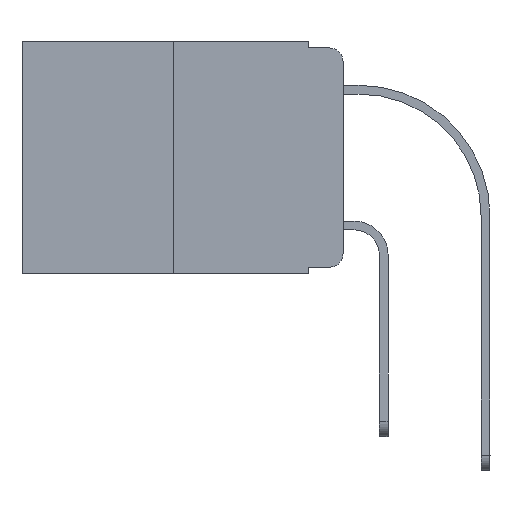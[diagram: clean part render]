
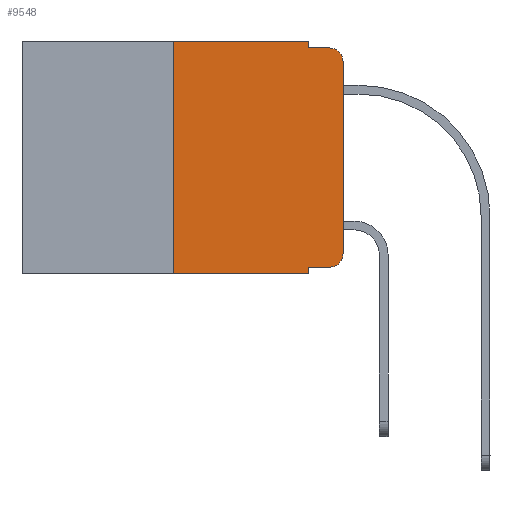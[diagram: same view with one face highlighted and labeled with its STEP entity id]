
A CAD part, left-side view. The second image highlights one B-rep face of the part: STEP entity #9548.
In plain terms, the highlighted planar face has unit normal (-1, 0, 0).
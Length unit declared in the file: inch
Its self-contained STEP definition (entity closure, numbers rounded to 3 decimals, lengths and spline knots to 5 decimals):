
#168 = CARTESIAN_POINT ( 'NONE',  ( 0., 0.02, -0.01 ) ) ;
#239 = VECTOR ( 'NONE', #13982, 39.37008 ) ;
#399 = DIRECTION ( 'NONE',  ( 0., -1., 0. ) ) ;
#440 = ORIENTED_EDGE ( 'NONE', *, *, #2540, .F. ) ;
#729 = EDGE_CURVE ( 'NONE', #20648, #1539, #17899, .T. ) ;
#860 = ORIENTED_EDGE ( 'NONE', *, *, #24218, .F. ) ;
#1041 = ORIENTED_EDGE ( 'NONE', *, *, #22903, .F. ) ;
#1135 = DIRECTION ( 'NONE',  ( 0., -1., 0. ) ) ;
#1462 = ORIENTED_EDGE ( 'NONE', *, *, #11914, .F. ) ;
#1539 = VERTEX_POINT ( 'NONE', #6256 ) ;
#2211 = CARTESIAN_POINT ( 'NONE',  ( 0., 0.051, 0. ) ) ;
#2469 = VECTOR ( 'NONE', #6436, 39.37008 ) ;
#2540 = EDGE_CURVE ( 'NONE', #20648, #21269, #13048, .T. ) ;
#2630 = LINE ( 'NONE', #10619, #2469 ) ;
#2850 = AXIS2_PLACEMENT_3D ( 'NONE', #13515, #21236, #13656 ) ;
#2889 = ORIENTED_EDGE ( 'NONE', *, *, #10489, .T. ) ;
#2893 = LINE ( 'NONE', #4797, #11804 ) ;
#3993 = CARTESIAN_POINT ( 'NONE',  ( 0., 0.25, -0.343 ) ) ;
#4261 = CARTESIAN_POINT ( 'NONE',  ( 0., 0.25, 0. ) ) ;
#4791 = DIRECTION ( 'NONE',  ( 0., 0., -1. ) ) ;
#4797 = CARTESIAN_POINT ( 'NONE',  ( 0., 0.051, -0.01 ) ) ;
#4845 = VERTEX_POINT ( 'NONE', #12068 ) ;
#5395 = LINE ( 'NONE', #16711, #6885 ) ;
#6146 = CIRCLE ( 'NONE', #2850, 0.02 ) ;
#6256 = CARTESIAN_POINT ( 'NONE',  ( 0., 0.02, -0.333 ) ) ;
#6436 = DIRECTION ( 'NONE',  ( 0., -1., 0. ) ) ;
#6885 = VECTOR ( 'NONE', #7432, 39.37008 ) ;
#7432 = DIRECTION ( 'NONE',  ( 0., -1., 0. ) ) ;
#7438 = CARTESIAN_POINT ( 'NONE',  ( 0., 0.25, 0. ) ) ;
#8888 = EDGE_CURVE ( 'NONE', #1539, #14236, #20594, .T. ) ;
#9020 = FACE_OUTER_BOUND ( 'NONE', #10609, .T. ) ;
#9548 = ADVANCED_FACE ( 'NONE', ( #9020 ), #20679, .F. ) ;
#9594 = VERTEX_POINT ( 'NONE', #14889 ) ;
#9600 = DIRECTION ( 'NONE',  ( 0., 0., 1. ) ) ;
#10489 = EDGE_CURVE ( 'NONE', #20383, #21269, #5395, .T. ) ;
#10609 = EDGE_LOOP ( 'NONE', ( #11493, #17040, #1041, #1462, #860, #23297, #2889, #440, #12570, #12920 ) ) ;
#10619 = CARTESIAN_POINT ( 'NONE',  ( 0., 0.473, 0. ) ) ;
#10762 = VERTEX_POINT ( 'NONE', #12007 ) ;
#11179 = CARTESIAN_POINT ( 'NONE',  ( 0., 0.051, -0.343 ) ) ;
#11493 = ORIENTED_EDGE ( 'NONE', *, *, #20991, .T. ) ;
#11804 = VECTOR ( 'NONE', #1135, 39.37008 ) ;
#11822 = CARTESIAN_POINT ( 'NONE',  ( 0., 0., 0. ) ) ;
#11863 = DIRECTION ( 'NONE',  ( -1., 0., 0. ) ) ;
#11914 = EDGE_CURVE ( 'NONE', #10762, #4845, #15546, .T. ) ;
#12007 = CARTESIAN_POINT ( 'NONE',  ( 0., 0.051, 0. ) ) ;
#12068 = CARTESIAN_POINT ( 'NONE',  ( 0., 0.051, -0.01 ) ) ;
#12185 = CARTESIAN_POINT ( 'NONE',  ( 0., 0.051, -0.333 ) ) ;
#12570 = ORIENTED_EDGE ( 'NONE', *, *, #729, .T. ) ;
#12920 = ORIENTED_EDGE ( 'NONE', *, *, #8888, .T. ) ;
#13048 = LINE ( 'NONE', #14845, #15300 ) ;
#13405 = LINE ( 'NONE', #7438, #22323 ) ;
#13515 = CARTESIAN_POINT ( 'NONE',  ( 0., 0.02, -0.03 ) ) ;
#13656 = DIRECTION ( 'NONE',  ( 0., 0., -1. ) ) ;
#13982 = DIRECTION ( 'NONE',  ( 0., 0., 1. ) ) ;
#14236 = VERTEX_POINT ( 'NONE', #16738 ) ;
#14682 = VERTEX_POINT ( 'NONE', #168 ) ;
#14845 = CARTESIAN_POINT ( 'NONE',  ( 0., 0.051, 0. ) ) ;
#14889 = CARTESIAN_POINT ( 'NONE',  ( 0., 0., -0.03 ) ) ;
#15300 = VECTOR ( 'NONE', #4791, 39.37008 ) ;
#15546 = LINE ( 'NONE', #2211, #19998 ) ;
#16711 = CARTESIAN_POINT ( 'NONE',  ( 0., 0.473, -0.343 ) ) ;
#16738 = CARTESIAN_POINT ( 'NONE',  ( 0., 0., -0.313 ) ) ;
#17040 = ORIENTED_EDGE ( 'NONE', *, *, #23680, .T. ) ;
#17714 = CARTESIAN_POINT ( 'NONE',  ( 0., 0.02, -0.313 ) ) ;
#17899 = LINE ( 'NONE', #12185, #24867 ) ;
#19243 = VERTEX_POINT ( 'NONE', #4261 ) ;
#19998 = VECTOR ( 'NONE', #23249, 39.37008 ) ;
#20383 = VERTEX_POINT ( 'NONE', #3993 ) ;
#20594 = CIRCLE ( 'NONE', #21000, 0.02 ) ;
#20648 = VERTEX_POINT ( 'NONE', #23744 ) ;
#20679 = PLANE ( 'NONE',  #21420 ) ;
#20991 = EDGE_CURVE ( 'NONE', #14236, #9594, #23464, .T. ) ;
#21000 = AXIS2_PLACEMENT_3D ( 'NONE', #17714, #11863, #23498 ) ;
#21057 = CARTESIAN_POINT ( 'NONE',  ( 0., 0.473, 0. ) ) ;
#21236 = DIRECTION ( 'NONE',  ( -1., 0., 0. ) ) ;
#21269 = VERTEX_POINT ( 'NONE', #11179 ) ;
#21420 = AXIS2_PLACEMENT_3D ( 'NONE', #21057, #24861, #24622 ) ;
#22323 = VECTOR ( 'NONE', #9600, 39.37008 ) ;
#22903 = EDGE_CURVE ( 'NONE', #4845, #14682, #2893, .T. ) ;
#23249 = DIRECTION ( 'NONE',  ( 0., 0., -1. ) ) ;
#23297 = ORIENTED_EDGE ( 'NONE', *, *, #24330, .F. ) ;
#23464 = LINE ( 'NONE', #11822, #239 ) ;
#23498 = DIRECTION ( 'NONE',  ( 0., 0., -1. ) ) ;
#23680 = EDGE_CURVE ( 'NONE', #9594, #14682, #6146, .T. ) ;
#23744 = CARTESIAN_POINT ( 'NONE',  ( 0., 0.051, -0.333 ) ) ;
#24218 = EDGE_CURVE ( 'NONE', #19243, #10762, #2630, .T. ) ;
#24330 = EDGE_CURVE ( 'NONE', #20383, #19243, #13405, .T. ) ;
#24622 = DIRECTION ( 'NONE',  ( 0., 0., -1. ) ) ;
#24861 = DIRECTION ( 'NONE',  ( 1., 0., 0. ) ) ;
#24867 = VECTOR ( 'NONE', #399, 39.37008 ) ;
